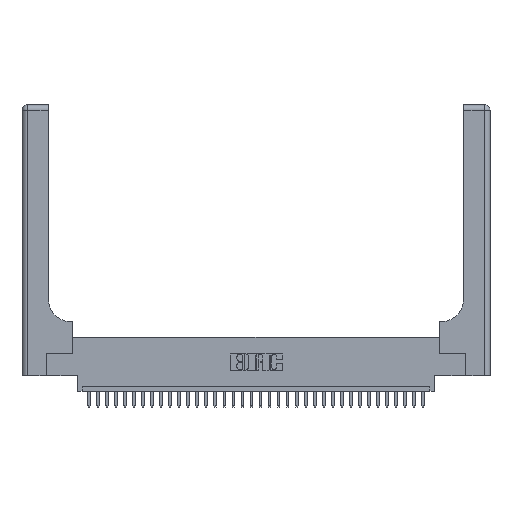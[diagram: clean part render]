
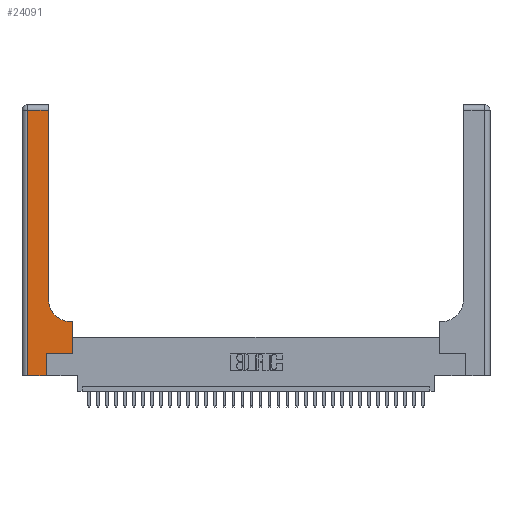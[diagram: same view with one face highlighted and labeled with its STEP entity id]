
A CAD part, top view. The second image highlights one B-rep face of the part: STEP entity #24091.
In plain terms, the highlighted planar face has unit normal (0, 0, 1).
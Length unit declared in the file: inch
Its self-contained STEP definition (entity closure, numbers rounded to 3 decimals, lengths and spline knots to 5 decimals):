
#83 = EDGE_CURVE ( 'NONE', #899, #33107, #28794, .T. ) ;
#486 = DIRECTION ( 'NONE',  ( 1., 0., 0. ) ) ;
#661 = VECTOR ( 'NONE', #486, 39.37008 ) ;
#899 = VERTEX_POINT ( 'NONE', #29102 ) ;
#1839 = DIRECTION ( 'NONE',  ( 1., 0., 0. ) ) ;
#1950 = LINE ( 'NONE', #32459, #661 ) ;
#2847 = VERTEX_POINT ( 'NONE', #29646 ) ;
#2945 = ORIENTED_EDGE ( 'NONE', *, *, #24089, .T. ) ;
#4111 = DIRECTION ( 'NONE',  ( 1., 0., 0. ) ) ;
#4237 = ORIENTED_EDGE ( 'NONE', *, *, #83, .T. ) ;
#4467 = VERTEX_POINT ( 'NONE', #21012 ) ;
#4608 = CARTESIAN_POINT ( 'NONE',  ( 0.269, 0.25, 0.37 ) ) ;
#6858 = CARTESIAN_POINT ( 'NONE',  ( 0.5415, 0.6, 0.37 ) ) ;
#7320 = LINE ( 'NONE', #28700, #20255 ) ;
#7476 = CARTESIAN_POINT ( 'NONE',  ( 0.06, 3., 0.37 ) ) ;
#7596 = CARTESIAN_POINT ( 'NONE',  ( 0.269, 0.25, 0.37 ) ) ;
#7627 = VECTOR ( 'NONE', #18827, 39.37008 ) ;
#8331 = EDGE_CURVE ( 'NONE', #19828, #16683, #20003, .T. ) ;
#8568 = CARTESIAN_POINT ( 'NONE',  ( 0.5585, 0.6, 0.37 ) ) ;
#8703 = DIRECTION ( 'NONE',  ( 0., 1., 0. ) ) ;
#9703 = DIRECTION ( 'NONE',  ( -1., 0., 0. ) ) ;
#10456 = ORIENTED_EDGE ( 'NONE', *, *, #8331, .T. ) ;
#10577 = FACE_OUTER_BOUND ( 'NONE', #13923, .T. ) ;
#10983 = CARTESIAN_POINT ( 'NONE',  ( 0.269, 0., 0.37 ) ) ;
#11805 = CARTESIAN_POINT ( 'NONE',  ( 0., 3., 0.37 ) ) ;
#12501 = CARTESIAN_POINT ( 'NONE',  ( 0.5415, 0.85, 0.37 ) ) ;
#13072 = LINE ( 'NONE', #10983, #7627 ) ;
#13875 = EDGE_CURVE ( 'NONE', #24201, #22865, #24493, .T. ) ;
#13923 = EDGE_LOOP ( 'NONE', ( #2945, #22394, #4237, #29096, #15228, #10456, #21246, #15312, #24940 ) ) ;
#14139 = EDGE_CURVE ( 'NONE', #33107, #2847, #1950, .T. ) ;
#14893 = CARTESIAN_POINT ( 'NONE',  ( 0.2915, 0.6, 0.37 ) ) ;
#15179 = DIRECTION ( 'NONE',  ( -1., 0., 0. ) ) ;
#15188 = CARTESIAN_POINT ( 'NONE',  ( 0.2915, 0.85, 0.37 ) ) ;
#15228 = ORIENTED_EDGE ( 'NONE', *, *, #30722, .T. ) ;
#15312 = ORIENTED_EDGE ( 'NONE', *, *, #13875, .T. ) ;
#15419 = CARTESIAN_POINT ( 'NONE',  ( 0.5585, 0.25, 0.37 ) ) ;
#15449 = VECTOR ( 'NONE', #27282, 39.37008 ) ;
#16650 = EDGE_CURVE ( 'NONE', #22865, #17735, #30008, .T. ) ;
#16683 = VERTEX_POINT ( 'NONE', #15419 ) ;
#17051 = AXIS2_PLACEMENT_3D ( 'NONE', #12501, #20077, #4111 ) ;
#17254 = VECTOR ( 'NONE', #32615, 39.37008 ) ;
#17735 = VERTEX_POINT ( 'NONE', #15188 ) ;
#18827 = DIRECTION ( 'NONE',  ( 0., 1., 0. ) ) ;
#19828 = VERTEX_POINT ( 'NONE', #7596 ) ;
#20003 = LINE ( 'NONE', #4608, #29645 ) ;
#20077 = DIRECTION ( 'NONE',  ( 0., 0., -1. ) ) ;
#20255 = VECTOR ( 'NONE', #15179, 39.37008 ) ;
#20341 = VECTOR ( 'NONE', #8703, 39.37008 ) ;
#21012 = CARTESIAN_POINT ( 'NONE',  ( 0.2915, 2.94, 0.37 ) ) ;
#21246 = ORIENTED_EDGE ( 'NONE', *, *, #27919, .T. ) ;
#22025 = LINE ( 'NONE', #24682, #20341 ) ;
#22394 = ORIENTED_EDGE ( 'NONE', *, *, #23168, .T. ) ;
#22815 = VECTOR ( 'NONE', #9703, 39.37008 ) ;
#22865 = VERTEX_POINT ( 'NONE', #6858 ) ;
#23168 = EDGE_CURVE ( 'NONE', #4467, #899, #7320, .T. ) ;
#23233 = AXIS2_PLACEMENT_3D ( 'NONE', #11805, #28381, #33525 ) ;
#24089 = EDGE_CURVE ( 'NONE', #17735, #4467, #31470, .T. ) ;
#24091 = ADVANCED_FACE ( 'NONE', ( #10577 ), #30275, .F. ) ;
#24201 = VERTEX_POINT ( 'NONE', #8568 ) ;
#24493 = LINE ( 'NONE', #14893, #22815 ) ;
#24682 = CARTESIAN_POINT ( 'NONE',  ( 0.5585, 0.25, 0.37 ) ) ;
#24940 = ORIENTED_EDGE ( 'NONE', *, *, #16650, .T. ) ;
#25673 = CARTESIAN_POINT ( 'NONE',  ( 0.06, 0., 0.37 ) ) ;
#27282 = DIRECTION ( 'NONE',  ( 0., -1., 0. ) ) ;
#27919 = EDGE_CURVE ( 'NONE', #16683, #24201, #22025, .T. ) ;
#28381 = DIRECTION ( 'NONE',  ( 0., 0., -1. ) ) ;
#28700 = CARTESIAN_POINT ( 'NONE',  ( 0., 2.94, 0.37 ) ) ;
#28794 = LINE ( 'NONE', #7476, #15449 ) ;
#29096 = ORIENTED_EDGE ( 'NONE', *, *, #14139, .T. ) ;
#29102 = CARTESIAN_POINT ( 'NONE',  ( 0.06, 2.94, 0.37 ) ) ;
#29645 = VECTOR ( 'NONE', #1839, 39.37008 ) ;
#29646 = CARTESIAN_POINT ( 'NONE',  ( 0.269, 0., 0.37 ) ) ;
#29932 = CARTESIAN_POINT ( 'NONE',  ( 0.2915, 3., 0.37 ) ) ;
#30008 = CIRCLE ( 'NONE', #17051, 0.25 ) ;
#30275 = PLANE ( 'NONE',  #23233 ) ;
#30722 = EDGE_CURVE ( 'NONE', #2847, #19828, #13072, .T. ) ;
#31470 = LINE ( 'NONE', #29932, #17254 ) ;
#32459 = CARTESIAN_POINT ( 'NONE',  ( 0., 0., 0.37 ) ) ;
#32615 = DIRECTION ( 'NONE',  ( 0., 1., 0. ) ) ;
#33107 = VERTEX_POINT ( 'NONE', #25673 ) ;
#33525 = DIRECTION ( 'NONE',  ( -1., 0., 0. ) ) ;
